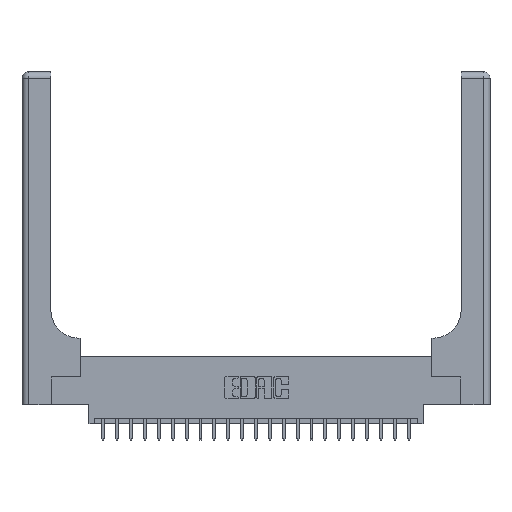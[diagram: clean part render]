
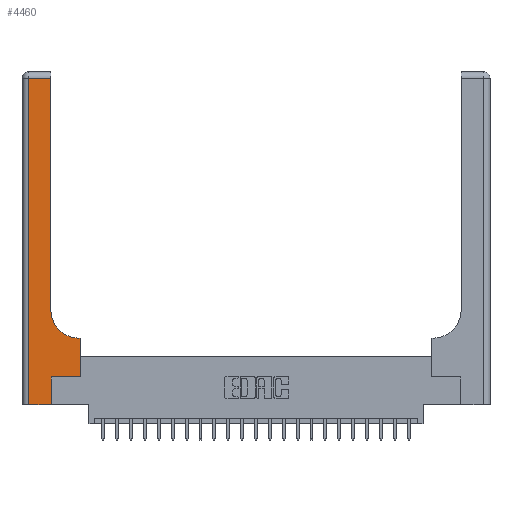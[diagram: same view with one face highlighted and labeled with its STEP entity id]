
A CAD part, top view. The second image highlights one B-rep face of the part: STEP entity #4460.
In plain terms, the highlighted planar face has unit normal (0, 0, 1).
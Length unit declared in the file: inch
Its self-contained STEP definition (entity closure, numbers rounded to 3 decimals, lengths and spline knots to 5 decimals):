
#593 = CARTESIAN_POINT ( 'NONE',  ( 0.528, 0.25, 0.37 ) ) ;
#1594 = VECTOR ( 'NONE', #14334, 39.37008 ) ;
#1808 = PLANE ( 'NONE',  #21160 ) ;
#2226 = VERTEX_POINT ( 'NONE', #15471 ) ;
#2386 = ORIENTED_EDGE ( 'NONE', *, *, #13295, .T. ) ;
#3104 = CARTESIAN_POINT ( 'NONE',  ( 0.265, 0., 0.37 ) ) ;
#3504 = ORIENTED_EDGE ( 'NONE', *, *, #3647, .T. ) ;
#3631 = ORIENTED_EDGE ( 'NONE', *, *, #7917, .T. ) ;
#3632 = DIRECTION ( 'NONE',  ( 0., 1., 0. ) ) ;
#3647 = EDGE_CURVE ( 'NONE', #4688, #8213, #20219, .T. ) ;
#3704 = CARTESIAN_POINT ( 'NONE',  ( 0.26, 2.94, 0.37 ) ) ;
#4316 = VERTEX_POINT ( 'NONE', #22643 ) ;
#4460 = ADVANCED_FACE ( 'NONE', ( #9521 ), #1808, .F. ) ;
#4688 = VERTEX_POINT ( 'NONE', #20212 ) ;
#4697 = DIRECTION ( 'NONE',  ( 0., 0., -1. ) ) ;
#4941 = DIRECTION ( 'NONE',  ( 0., 1., 0. ) ) ;
#5109 = LINE ( 'NONE', #14306, #14079 ) ;
#5354 = EDGE_LOOP ( 'NONE', ( #2386, #11043, #22720, #17983, #10210, #3504, #21167, #11729, #3631 ) ) ;
#5380 = DIRECTION ( 'NONE',  ( -1., 0., 0. ) ) ;
#5526 = CIRCLE ( 'NONE', #6169, 0.25 ) ;
#5666 = VECTOR ( 'NONE', #6206, 39.37008 ) ;
#6169 = AXIS2_PLACEMENT_3D ( 'NONE', #15424, #4697, #17157 ) ;
#6206 = DIRECTION ( 'NONE',  ( 0., -1., 0. ) ) ;
#6808 = LINE ( 'NONE', #9305, #15696 ) ;
#7155 = CARTESIAN_POINT ( 'NONE',  ( 0.26, 0.85, 0.37 ) ) ;
#7212 = VERTEX_POINT ( 'NONE', #18771 ) ;
#7356 = DIRECTION ( 'NONE',  ( -1., 0., 0. ) ) ;
#7917 = EDGE_CURVE ( 'NONE', #21340, #16865, #5526, .T. ) ;
#8213 = VERTEX_POINT ( 'NONE', #593 ) ;
#9305 = CARTESIAN_POINT ( 'NONE',  ( 0.26, 0.6, 0.37 ) ) ;
#9521 = FACE_OUTER_BOUND ( 'NONE', #5354, .T. ) ;
#9560 = LINE ( 'NONE', #14263, #1594 ) ;
#10210 = ORIENTED_EDGE ( 'NONE', *, *, #12637, .T. ) ;
#10575 = EDGE_CURVE ( 'NONE', #21395, #2226, #5109, .T. ) ;
#10680 = CARTESIAN_POINT ( 'NONE',  ( 0.51, 0.6, 0.37 ) ) ;
#10691 = LINE ( 'NONE', #11837, #11243 ) ;
#11043 = ORIENTED_EDGE ( 'NONE', *, *, #10575, .T. ) ;
#11076 = DIRECTION ( 'NONE',  ( -1., 0., 0. ) ) ;
#11191 = VECTOR ( 'NONE', #4941, 39.37008 ) ;
#11243 = VECTOR ( 'NONE', #18871, 39.37008 ) ;
#11406 = EDGE_CURVE ( 'NONE', #7212, #21340, #6808, .T. ) ;
#11678 = EDGE_CURVE ( 'NONE', #19371, #4316, #10691, .T. ) ;
#11729 = ORIENTED_EDGE ( 'NONE', *, *, #11406, .T. ) ;
#11837 = CARTESIAN_POINT ( 'NONE',  ( 0., 0., 0.37 ) ) ;
#12419 = CARTESIAN_POINT ( 'NONE',  ( 0.06, 0., 0.37 ) ) ;
#12637 = EDGE_CURVE ( 'NONE', #4316, #4688, #19392, .T. ) ;
#13295 = EDGE_CURVE ( 'NONE', #16865, #21395, #16131, .T. ) ;
#14079 = VECTOR ( 'NONE', #5380, 39.37008 ) ;
#14263 = CARTESIAN_POINT ( 'NONE',  ( 0.528, 0.25, 0.37 ) ) ;
#14306 = CARTESIAN_POINT ( 'NONE',  ( 0., 2.94, 0.37 ) ) ;
#14334 = DIRECTION ( 'NONE',  ( 0., 1., 0. ) ) ;
#14418 = CARTESIAN_POINT ( 'NONE',  ( 0., 3., 0.37 ) ) ;
#14621 = LINE ( 'NONE', #21974, #5666 ) ;
#15098 = VECTOR ( 'NONE', #22748, 39.37008 ) ;
#15424 = CARTESIAN_POINT ( 'NONE',  ( 0.51, 0.85, 0.37 ) ) ;
#15471 = CARTESIAN_POINT ( 'NONE',  ( 0.06, 2.94, 0.37 ) ) ;
#15696 = VECTOR ( 'NONE', #11076, 39.37008 ) ;
#16131 = LINE ( 'NONE', #16158, #21252 ) ;
#16158 = CARTESIAN_POINT ( 'NONE',  ( 0.26, 3., 0.37 ) ) ;
#16865 = VERTEX_POINT ( 'NONE', #7155 ) ;
#17157 = DIRECTION ( 'NONE',  ( 1., 0., 0. ) ) ;
#17497 = EDGE_CURVE ( 'NONE', #8213, #7212, #9560, .T. ) ;
#17902 = DIRECTION ( 'NONE',  ( 0., 0., -1. ) ) ;
#17983 = ORIENTED_EDGE ( 'NONE', *, *, #11678, .T. ) ;
#18771 = CARTESIAN_POINT ( 'NONE',  ( 0.528, 0.6, 0.37 ) ) ;
#18871 = DIRECTION ( 'NONE',  ( 1., 0., 0. ) ) ;
#19371 = VERTEX_POINT ( 'NONE', #12419 ) ;
#19392 = LINE ( 'NONE', #3104, #11191 ) ;
#20212 = CARTESIAN_POINT ( 'NONE',  ( 0.265, 0.25, 0.37 ) ) ;
#20219 = LINE ( 'NONE', #21082, #15098 ) ;
#20267 = EDGE_CURVE ( 'NONE', #2226, #19371, #14621, .T. ) ;
#21082 = CARTESIAN_POINT ( 'NONE',  ( 0.265, 0.25, 0.37 ) ) ;
#21160 = AXIS2_PLACEMENT_3D ( 'NONE', #14418, #17902, #7356 ) ;
#21167 = ORIENTED_EDGE ( 'NONE', *, *, #17497, .T. ) ;
#21252 = VECTOR ( 'NONE', #3632, 39.37008 ) ;
#21340 = VERTEX_POINT ( 'NONE', #10680 ) ;
#21395 = VERTEX_POINT ( 'NONE', #3704 ) ;
#21974 = CARTESIAN_POINT ( 'NONE',  ( 0.06, 3., 0.37 ) ) ;
#22643 = CARTESIAN_POINT ( 'NONE',  ( 0.265, 0., 0.37 ) ) ;
#22720 = ORIENTED_EDGE ( 'NONE', *, *, #20267, .T. ) ;
#22748 = DIRECTION ( 'NONE',  ( 1., 0., 0. ) ) ;
